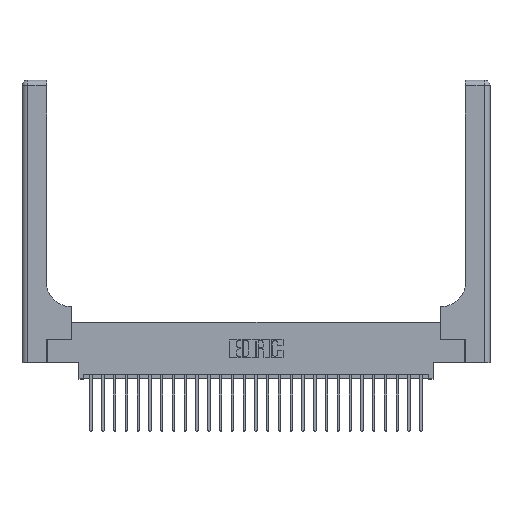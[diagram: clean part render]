
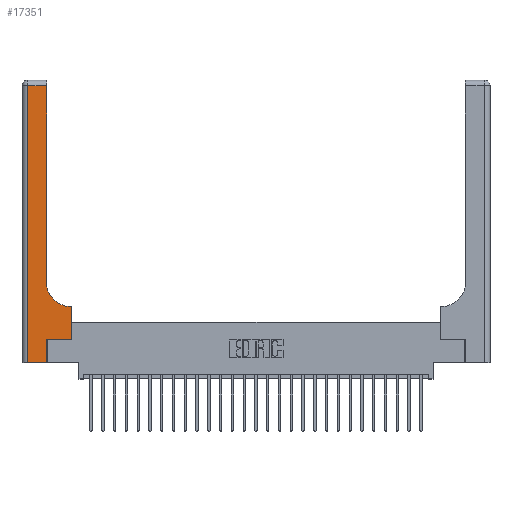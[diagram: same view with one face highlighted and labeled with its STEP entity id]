
A CAD part, top view. The second image highlights one B-rep face of the part: STEP entity #17351.
In plain terms, the highlighted planar face has unit normal (0, 0, 1).
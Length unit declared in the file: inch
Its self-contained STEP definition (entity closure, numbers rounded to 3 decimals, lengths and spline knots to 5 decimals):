
#173 = EDGE_CURVE ( 'NONE', #5774, #12686, #17834, .T. ) ;
#186 = CARTESIAN_POINT ( 'NONE',  ( 0., 3., 0.37 ) ) ;
#486 = VERTEX_POINT ( 'NONE', #6835 ) ;
#582 = PLANE ( 'NONE',  #19909 ) ;
#645 = VECTOR ( 'NONE', #1268, 39.37008 ) ;
#752 = ORIENTED_EDGE ( 'NONE', *, *, #5836, .T. ) ;
#794 = VERTEX_POINT ( 'NONE', #1542 ) ;
#996 = CARTESIAN_POINT ( 'NONE',  ( 0.26, 3., 0.37 ) ) ;
#1268 = DIRECTION ( 'NONE',  ( 0., 1., 0. ) ) ;
#1542 = CARTESIAN_POINT ( 'NONE',  ( 0.528, 0.6, 0.37 ) ) ;
#1647 = CARTESIAN_POINT ( 'NONE',  ( 0.06, 0., 0.37 ) ) ;
#1730 = DIRECTION ( 'NONE',  ( -1., 0., 0. ) ) ;
#2078 = VERTEX_POINT ( 'NONE', #5832 ) ;
#2863 = LINE ( 'NONE', #9009, #9353 ) ;
#2999 = DIRECTION ( 'NONE',  ( 0., 0., -1. ) ) ;
#3319 = VECTOR ( 'NONE', #13352, 39.37008 ) ;
#3404 = VECTOR ( 'NONE', #5134, 39.37008 ) ;
#3500 = ORIENTED_EDGE ( 'NONE', *, *, #173, .T. ) ;
#3650 = CARTESIAN_POINT ( 'NONE',  ( 0.528, 0.25, 0.37 ) ) ;
#3899 = CARTESIAN_POINT ( 'NONE',  ( 0.265, 0.25, 0.37 ) ) ;
#3965 = DIRECTION ( 'NONE',  ( 0., 1., 0. ) ) ;
#4133 = CARTESIAN_POINT ( 'NONE',  ( 0.06, 2.94, 0.37 ) ) ;
#4865 = CARTESIAN_POINT ( 'NONE',  ( 0.26, 2.94, 0.37 ) ) ;
#5027 = ORIENTED_EDGE ( 'NONE', *, *, #18028, .T. ) ;
#5134 = DIRECTION ( 'NONE',  ( 0., 1., 0. ) ) ;
#5774 = VERTEX_POINT ( 'NONE', #4865 ) ;
#5832 = CARTESIAN_POINT ( 'NONE',  ( 0.26, 0.85, 0.37 ) ) ;
#5836 = EDGE_CURVE ( 'NONE', #2078, #5774, #19331, .T. ) ;
#6247 = VERTEX_POINT ( 'NONE', #8843 ) ;
#6327 = DIRECTION ( 'NONE',  ( 0., 0., -1. ) ) ;
#6585 = EDGE_CURVE ( 'NONE', #6247, #8759, #24059, .T. ) ;
#6835 = CARTESIAN_POINT ( 'NONE',  ( 0.51, 0.6, 0.37 ) ) ;
#6963 = ORIENTED_EDGE ( 'NONE', *, *, #6585, .T. ) ;
#7636 = DIRECTION ( 'NONE',  ( -1., 0., 0. ) ) ;
#7732 = CARTESIAN_POINT ( 'NONE',  ( 0.26, 0.6, 0.37 ) ) ;
#8059 = ORIENTED_EDGE ( 'NONE', *, *, #14779, .T. ) ;
#8759 = VERTEX_POINT ( 'NONE', #3899 ) ;
#8843 = CARTESIAN_POINT ( 'NONE',  ( 0.265, 0., 0.37 ) ) ;
#8853 = VERTEX_POINT ( 'NONE', #1647 ) ;
#9009 = CARTESIAN_POINT ( 'NONE',  ( 0.06, 3., 0.37 ) ) ;
#9200 = VERTEX_POINT ( 'NONE', #17815 ) ;
#9353 = VECTOR ( 'NONE', #21197, 39.37008 ) ;
#9356 = LINE ( 'NONE', #7732, #22484 ) ;
#9728 = CARTESIAN_POINT ( 'NONE',  ( 0.265, 0., 0.37 ) ) ;
#10229 = VECTOR ( 'NONE', #3965, 39.37008 ) ;
#10449 = VECTOR ( 'NONE', #7636, 39.37008 ) ;
#10610 = DIRECTION ( 'NONE',  ( -1., 0., 0. ) ) ;
#11201 = CARTESIAN_POINT ( 'NONE',  ( 0.265, 0.25, 0.37 ) ) ;
#11249 = VECTOR ( 'NONE', #15950, 39.37008 ) ;
#11915 = CARTESIAN_POINT ( 'NONE',  ( 0., 0., 0.37 ) ) ;
#12428 = EDGE_CURVE ( 'NONE', #8853, #6247, #13675, .T. ) ;
#12686 = VERTEX_POINT ( 'NONE', #4133 ) ;
#12814 = LINE ( 'NONE', #11201, #3319 ) ;
#13352 = DIRECTION ( 'NONE',  ( 1., 0., 0. ) ) ;
#13460 = LINE ( 'NONE', #3650, #645 ) ;
#13675 = LINE ( 'NONE', #11915, #11249 ) ;
#14779 = EDGE_CURVE ( 'NONE', #9200, #794, #13460, .T. ) ;
#15950 = DIRECTION ( 'NONE',  ( 1., 0., 0. ) ) ;
#17073 = DIRECTION ( 'NONE',  ( 1., 0., 0. ) ) ;
#17145 = EDGE_LOOP ( 'NONE', ( #752, #3500, #22210, #23970, #6963, #26308, #8059, #5027, #23707 ) ) ;
#17351 = ADVANCED_FACE ( 'NONE', ( #24817 ), #582, .F. ) ;
#17815 = CARTESIAN_POINT ( 'NONE',  ( 0.528, 0.25, 0.37 ) ) ;
#17834 = LINE ( 'NONE', #26008, #10449 ) ;
#18028 = EDGE_CURVE ( 'NONE', #794, #486, #9356, .T. ) ;
#18746 = CIRCLE ( 'NONE', #20022, 0.25 ) ;
#19331 = LINE ( 'NONE', #996, #3404 ) ;
#19909 = AXIS2_PLACEMENT_3D ( 'NONE', #186, #6327, #10610 ) ;
#20022 = AXIS2_PLACEMENT_3D ( 'NONE', #21333, #2999, #17073 ) ;
#20218 = EDGE_CURVE ( 'NONE', #8759, #9200, #12814, .T. ) ;
#20638 = EDGE_CURVE ( 'NONE', #486, #2078, #18746, .T. ) ;
#21197 = DIRECTION ( 'NONE',  ( 0., -1., 0. ) ) ;
#21333 = CARTESIAN_POINT ( 'NONE',  ( 0.51, 0.85, 0.37 ) ) ;
#22210 = ORIENTED_EDGE ( 'NONE', *, *, #25870, .T. ) ;
#22484 = VECTOR ( 'NONE', #1730, 39.37008 ) ;
#23707 = ORIENTED_EDGE ( 'NONE', *, *, #20638, .T. ) ;
#23970 = ORIENTED_EDGE ( 'NONE', *, *, #12428, .T. ) ;
#24059 = LINE ( 'NONE', #9728, #10229 ) ;
#24817 = FACE_OUTER_BOUND ( 'NONE', #17145, .T. ) ;
#25870 = EDGE_CURVE ( 'NONE', #12686, #8853, #2863, .T. ) ;
#26008 = CARTESIAN_POINT ( 'NONE',  ( 0., 2.94, 0.37 ) ) ;
#26308 = ORIENTED_EDGE ( 'NONE', *, *, #20218, .T. ) ;
